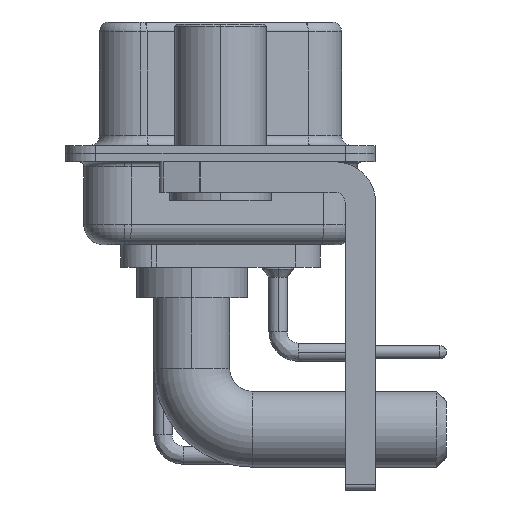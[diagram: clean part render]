
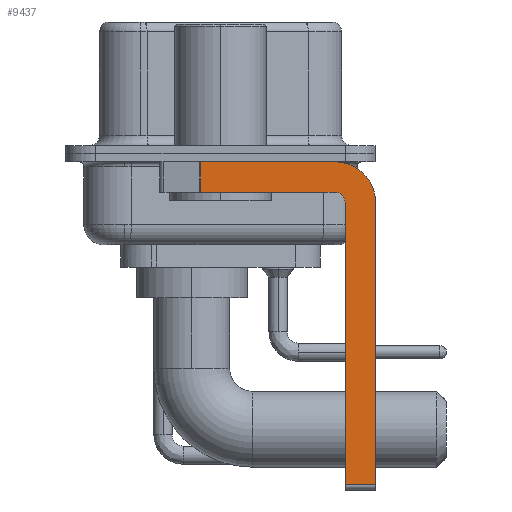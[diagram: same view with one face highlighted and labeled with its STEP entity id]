
A CAD part, left-side view. The second image highlights one B-rep face of the part: STEP entity #9437.
In plain terms, the highlighted planar face has unit normal (-1, 0, 0).
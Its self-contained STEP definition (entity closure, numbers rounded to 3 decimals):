
#282 = ORIENTED_EDGE ( 'NONE', *, *, #30134, .F. ) ;
#983 = VERTEX_POINT ( 'NONE', #6875 ) ;
#2041 = VECTOR ( 'NONE', #4162, 1000. ) ;
#2071 = DIRECTION ( 'NONE',  ( 1., 0., 0. ) ) ;
#2327 = CARTESIAN_POINT ( 'NONE',  ( -2.9, -5.65, -1.9 ) ) ;
#2785 = VERTEX_POINT ( 'NONE', #15537 ) ;
#3117 = VECTOR ( 'NONE', #36174, 1000. ) ;
#3754 = ORIENTED_EDGE ( 'NONE', *, *, #23819, .F. ) ;
#4162 = DIRECTION ( 'NONE',  ( 0., -1., 0. ) ) ;
#5185 = EDGE_CURVE ( 'NONE', #983, #22658, #29897, .T. ) ;
#5229 = LINE ( 'NONE', #36266, #6951 ) ;
#5491 = VERTEX_POINT ( 'NONE', #28644 ) ;
#6627 = VECTOR ( 'NONE', #21268, 1000. ) ;
#6875 = CARTESIAN_POINT ( 'NONE',  ( -2.9, -5.65, -0.4 ) ) ;
#6951 = VECTOR ( 'NONE', #28284, 1000. ) ;
#7840 = CARTESIAN_POINT ( 'NONE',  ( -2.9, -5.65, -2.4 ) ) ;
#9437 = ADVANCED_FACE ( 'NONE', ( #29287 ), #9767, .F. ) ;
#9767 = PLANE ( 'NONE',  #20668 ) ;
#11666 = CARTESIAN_POINT ( 'NONE',  ( -2.9, -6.15, -16.35 ) ) ;
#12082 = AXIS2_PLACEMENT_3D ( 'NONE', #7840, #2071, #13420 ) ;
#13399 = VECTOR ( 'NONE', #27481, 1000. ) ;
#13420 = DIRECTION ( 'NONE',  ( 0., 0., -1. ) ) ;
#13489 = DIRECTION ( 'NONE',  ( -1., 0., 0. ) ) ;
#13850 = VERTEX_POINT ( 'NONE', #11666 ) ;
#14444 = EDGE_CURVE ( 'NONE', #2785, #983, #29451, .T. ) ;
#14621 = DIRECTION ( 'NONE',  ( 1., 0., 0. ) ) ;
#15199 = CARTESIAN_POINT ( 'NONE',  ( -2.9, -7.65, -2.4 ) ) ;
#15537 = CARTESIAN_POINT ( 'NONE',  ( -2.9, 0.978, -0.4 ) ) ;
#15794 = EDGE_CURVE ( 'NONE', #2785, #31440, #24313, .T. ) ;
#16655 = DIRECTION ( 'NONE',  ( 0., 1., 0. ) ) ;
#16679 = ORIENTED_EDGE ( 'NONE', *, *, #5185, .F. ) ;
#17783 = DIRECTION ( 'NONE',  ( 0., 0., -1. ) ) ;
#19072 = CARTESIAN_POINT ( 'NONE',  ( -2.9, -7.65, -16.35 ) ) ;
#19075 = CARTESIAN_POINT ( 'NONE',  ( -2.9, -5.65, -2.4 ) ) ;
#20268 = CIRCLE ( 'NONE', #33329, 0.5 ) ;
#20650 = EDGE_LOOP ( 'NONE', ( #24243, #20951, #22973, #30976, #3754, #35270, #282, #16679 ) ) ;
#20668 = AXIS2_PLACEMENT_3D ( 'NONE', #28917, #14621, #17783 ) ;
#20951 = ORIENTED_EDGE ( 'NONE', *, *, #15794, .T. ) ;
#21266 = CARTESIAN_POINT ( 'NONE',  ( -2.9, 3., -0.4 ) ) ;
#21268 = DIRECTION ( 'NONE',  ( 0., -1., 0. ) ) ;
#21475 = VERTEX_POINT ( 'NONE', #19072 ) ;
#22546 = CARTESIAN_POINT ( 'NONE',  ( -2.9, -6.15, -2.4 ) ) ;
#22658 = VERTEX_POINT ( 'NONE', #15199 ) ;
#22726 = EDGE_CURVE ( 'NONE', #32906, #5491, #20268, .T. ) ;
#22973 = ORIENTED_EDGE ( 'NONE', *, *, #33750, .F. ) ;
#23819 = EDGE_CURVE ( 'NONE', #13850, #32906, #24840, .T. ) ;
#24150 = CARTESIAN_POINT ( 'NONE',  ( -2.9, -6.15, -16.6 ) ) ;
#24243 = ORIENTED_EDGE ( 'NONE', *, *, #14444, .F. ) ;
#24313 = LINE ( 'NONE', #30271, #13399 ) ;
#24840 = LINE ( 'NONE', #24150, #3117 ) ;
#26844 = CARTESIAN_POINT ( 'NONE',  ( -2.9, -5.65, -16.35 ) ) ;
#27481 = DIRECTION ( 'NONE',  ( 0., 0., -1. ) ) ;
#27614 = DIRECTION ( 'NONE',  ( 0., 0., 1. ) ) ;
#28284 = DIRECTION ( 'NONE',  ( 0., 0., -1. ) ) ;
#28644 = CARTESIAN_POINT ( 'NONE',  ( -2.9, -5.65, -1.9 ) ) ;
#28917 = CARTESIAN_POINT ( 'NONE',  ( -2.9, -5.65, -2.4 ) ) ;
#29287 = FACE_OUTER_BOUND ( 'NONE', #20650, .T. ) ;
#29451 = LINE ( 'NONE', #21266, #2041 ) ;
#29897 = CIRCLE ( 'NONE', #12082, 2. ) ;
#30134 = EDGE_CURVE ( 'NONE', #22658, #21475, #5229, .T. ) ;
#30184 = LINE ( 'NONE', #26844, #6627 ) ;
#30271 = CARTESIAN_POINT ( 'NONE',  ( -2.9, 0.978, -1.9 ) ) ;
#30591 = LINE ( 'NONE', #2327, #32669 ) ;
#30976 = ORIENTED_EDGE ( 'NONE', *, *, #22726, .F. ) ;
#31440 = VERTEX_POINT ( 'NONE', #33994 ) ;
#32669 = VECTOR ( 'NONE', #16655, 1000. ) ;
#32906 = VERTEX_POINT ( 'NONE', #22546 ) ;
#33329 = AXIS2_PLACEMENT_3D ( 'NONE', #19075, #13489, #27614 ) ;
#33750 = EDGE_CURVE ( 'NONE', #5491, #31440, #30591, .T. ) ;
#33994 = CARTESIAN_POINT ( 'NONE',  ( -2.9, 0.978, -1.9 ) ) ;
#35141 = EDGE_CURVE ( 'NONE', #13850, #21475, #30184, .T. ) ;
#35270 = ORIENTED_EDGE ( 'NONE', *, *, #35141, .T. ) ;
#36174 = DIRECTION ( 'NONE',  ( 0., 0., 1. ) ) ;
#36266 = CARTESIAN_POINT ( 'NONE',  ( -2.9, -7.65, -2.4 ) ) ;
